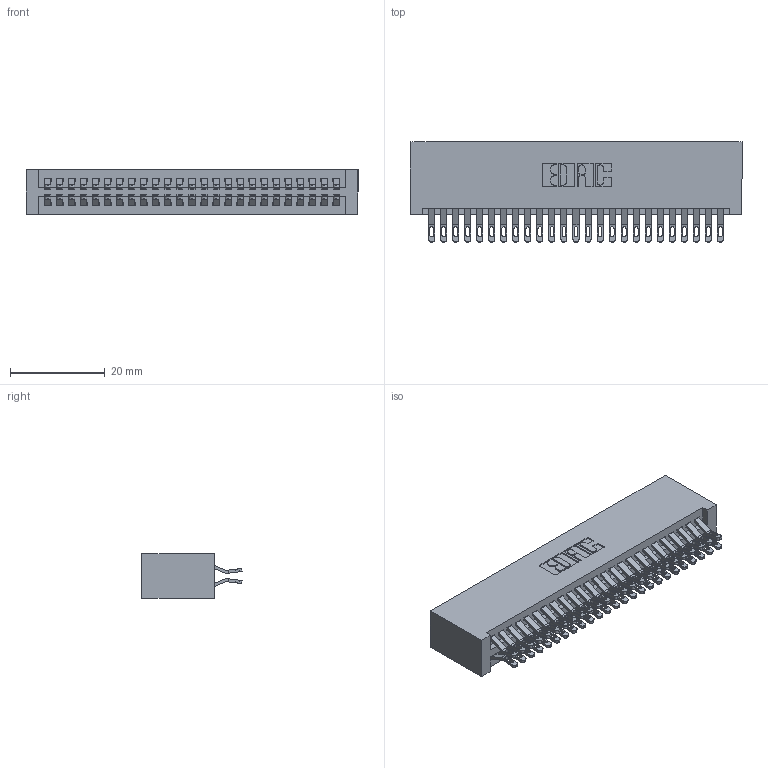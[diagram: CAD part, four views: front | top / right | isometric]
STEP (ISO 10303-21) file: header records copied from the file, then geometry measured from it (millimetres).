
FILE_DESCRIPTION (( 'STEP AP203' ), '1' );
FILE_NAME ('345-050-555-201.STEP', '2018-09-14T09:08:21', ( '' ), ( '' ), 'SwSTEP 2.0', 'SolidWorks 2016', '' );
FILE_SCHEMA (( 'CONFIG_CONTROL_DESIGN' ));
Length unit declared in the file: inch
Products named in the file (3): 345-292-001_555 Tail; 345-050-555-201; 345 Part_No Mounting Lugs
Assembly tree (51 placements, depth 2):
  345-050-555-201
    345 Part_No Mounting Lugs
    345-292-001_555 Tail  x50
Bounding box: 70.1 x 21.13 x 9.4 mm (x, y, z)
Volume: 7413.1 mm3; surface area: 11436.3 mm2
Topology: 51 solids, 51 shells, 2918 faces, 9167 edges, 6110 vertices
Faces by surface type: plane 1626, cylinder 1292
Entity records: 21953 total; most frequent: CARTESIAN_POINT 3730, ORIENTED_EDGE 3634, DIRECTION 3273, EDGE_CURVE 1817, LINE 1573, VECTOR 1573, VERTEX_POINT 1210, AXIS2_PLACEMENT_3D 850
